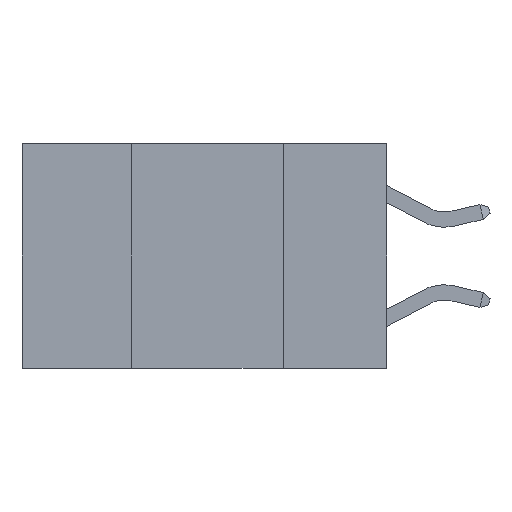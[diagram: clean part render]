
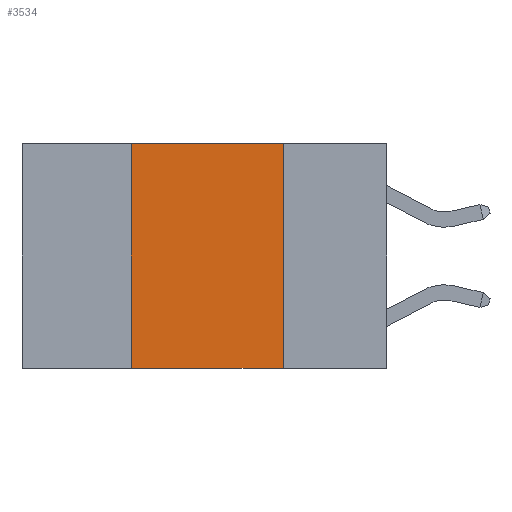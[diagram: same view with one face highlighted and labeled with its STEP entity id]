
A CAD part, left-side view. The second image highlights one B-rep face of the part: STEP entity #3534.
In plain terms, the highlighted planar face has unit normal (-1, 0, 0).
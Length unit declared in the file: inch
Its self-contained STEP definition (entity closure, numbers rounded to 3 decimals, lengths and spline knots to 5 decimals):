
#465 = DIRECTION ( 'NONE',  ( 0., -1., 0. ) ) ;
#915 = ORIENTED_EDGE ( 'NONE', *, *, #4023, .T. ) ;
#1136 = DIRECTION ( 'NONE',  ( 0., -1., 0. ) ) ;
#2942 = ORIENTED_EDGE ( 'NONE', *, *, #10916, .F. ) ;
#3006 = LINE ( 'NONE', #6504, #6859 ) ;
#3289 = VERTEX_POINT ( 'NONE', #10310 ) ;
#3318 = EDGE_LOOP ( 'NONE', ( #2942, #5374, #3939, #915 ) ) ;
#3456 = PLANE ( 'NONE',  #4969 ) ;
#3534 = ADVANCED_FACE ( 'NONE', ( #5508 ), #3456, .F. ) ;
#3640 = CARTESIAN_POINT ( 'NONE',  ( 0., 0.6, 0. ) ) ;
#3747 = VECTOR ( 'NONE', #8095, 39.37008 ) ;
#3939 = ORIENTED_EDGE ( 'NONE', *, *, #4396, .F. ) ;
#4023 = EDGE_CURVE ( 'NONE', #7518, #10065, #3006, .T. ) ;
#4251 = CARTESIAN_POINT ( 'NONE',  ( 0., 0.6, 0. ) ) ;
#4396 = EDGE_CURVE ( 'NONE', #7518, #10372, #9199, .T. ) ;
#4494 = CARTESIAN_POINT ( 'NONE',  ( 0., 0.42, 0. ) ) ;
#4969 = AXIS2_PLACEMENT_3D ( 'NONE', #3640, #10783, #10906 ) ;
#5374 = ORIENTED_EDGE ( 'NONE', *, *, #8590, .F. ) ;
#5508 = FACE_OUTER_BOUND ( 'NONE', #3318, .T. ) ;
#6353 = CARTESIAN_POINT ( 'NONE',  ( 0., 0.17, 0. ) ) ;
#6504 = CARTESIAN_POINT ( 'NONE',  ( 0., 0.6, -0.37 ) ) ;
#6859 = VECTOR ( 'NONE', #1136, 39.37008 ) ;
#6958 = LINE ( 'NONE', #4251, #7163 ) ;
#7163 = VECTOR ( 'NONE', #465, 39.37008 ) ;
#7417 = CARTESIAN_POINT ( 'NONE',  ( 0., 0.42, 0. ) ) ;
#7434 = VECTOR ( 'NONE', #9249, 39.37008 ) ;
#7518 = VERTEX_POINT ( 'NONE', #11036 ) ;
#8095 = DIRECTION ( 'NONE',  ( 0., 0., -1. ) ) ;
#8590 = EDGE_CURVE ( 'NONE', #10372, #3289, #6958, .T. ) ;
#9199 = LINE ( 'NONE', #4494, #7434 ) ;
#9249 = DIRECTION ( 'NONE',  ( 0., 0., 1. ) ) ;
#10019 = LINE ( 'NONE', #6353, #3747 ) ;
#10065 = VERTEX_POINT ( 'NONE', #10503 ) ;
#10310 = CARTESIAN_POINT ( 'NONE',  ( 0., 0.17, 0. ) ) ;
#10372 = VERTEX_POINT ( 'NONE', #7417 ) ;
#10503 = CARTESIAN_POINT ( 'NONE',  ( 0., 0.17, -0.37 ) ) ;
#10783 = DIRECTION ( 'NONE',  ( 1., 0., 0. ) ) ;
#10906 = DIRECTION ( 'NONE',  ( 0., 0., -1. ) ) ;
#10916 = EDGE_CURVE ( 'NONE', #3289, #10065, #10019, .T. ) ;
#11036 = CARTESIAN_POINT ( 'NONE',  ( 0., 0.42, -0.37 ) ) ;
